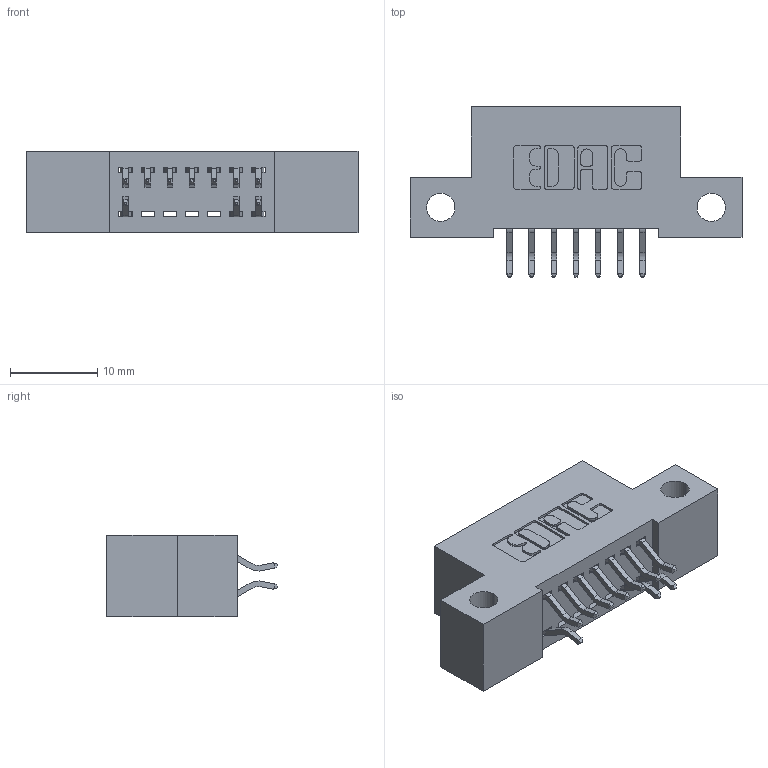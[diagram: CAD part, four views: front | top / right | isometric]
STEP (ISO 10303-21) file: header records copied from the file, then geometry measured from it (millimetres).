
FILE_DESCRIPTION (( 'STEP AP203' ), '1' );
FILE_NAME ('392-014-556-212.STEP', '2018-08-15T00:22:56', ( '' ), ( '' ), 'SwSTEP 2.0', 'SolidWorks 2016', '' );
FILE_SCHEMA (( 'CONFIG_CONTROL_DESIGN' ));
Length unit declared in the file: inch
Products named in the file (3): 342 Part_Side Mount; 345-292-001_556 Tail; 392-014-556-212
Assembly tree (11 placements, depth 2):
  392-014-556-212
    342 Part_Side Mount
    345-292-001_556 Tail  x10
Bounding box: 38.1 x 19.58 x 9.4 mm (x, y, z)
Volume: 3147.4 mm3; surface area: 3892.4 mm2
Topology: 11 solids, 11 shells, 714 faces, 2113 edges, 1394 vertices
Faces by surface type: plane 490, cylinder 224
Entity records: 8993 total; most frequent: CARTESIAN_POINT 1562, ORIENTED_EDGE 1490, DIRECTION 1381, EDGE_CURVE 745, LINE 609, VECTOR 609, VERTEX_POINT 494, AXIS2_PLACEMENT_3D 386
